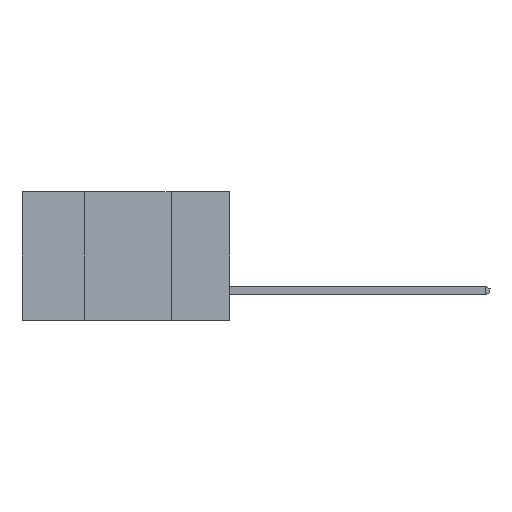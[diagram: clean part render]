
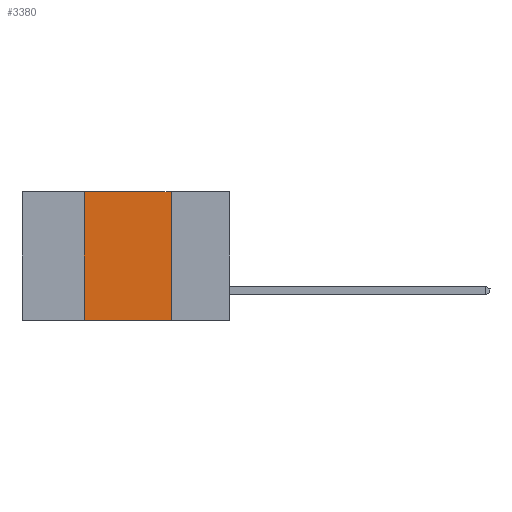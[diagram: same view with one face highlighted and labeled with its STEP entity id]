
A CAD part, left-side view. The second image highlights one B-rep face of the part: STEP entity #3380.
In plain terms, the highlighted planar face has unit normal (-1, 0, 0).
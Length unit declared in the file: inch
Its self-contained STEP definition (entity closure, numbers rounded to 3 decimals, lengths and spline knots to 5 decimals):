
#35 = CARTESIAN_POINT ( 'NONE',  ( 0., 0.42, -0.37 ) ) ;
#227 = ORIENTED_EDGE ( 'NONE', *, *, #5666, .F. ) ;
#707 = DIRECTION ( 'NONE',  ( 0., 0., -1. ) ) ;
#739 = AXIS2_PLACEMENT_3D ( 'NONE', #8256, #2847, #9026 ) ;
#811 = DIRECTION ( 'NONE',  ( 0., -1., 0. ) ) ;
#896 = CARTESIAN_POINT ( 'NONE',  ( 0., 0.17, -0.37 ) ) ;
#1425 = LINE ( 'NONE', #6782, #7478 ) ;
#2050 = ORIENTED_EDGE ( 'NONE', *, *, #7168, .F. ) ;
#2222 = EDGE_CURVE ( 'NONE', #7654, #8650, #4443, .T. ) ;
#2847 = DIRECTION ( 'NONE',  ( 1., 0., 0. ) ) ;
#3380 = ADVANCED_FACE ( 'NONE', ( #6602 ), #8207, .F. ) ;
#4443 = LINE ( 'NONE', #9164, #8667 ) ;
#4471 = DIRECTION ( 'NONE',  ( 0., 0., 1. ) ) ;
#5181 = EDGE_CURVE ( 'NONE', #6304, #8650, #1425, .T. ) ;
#5288 = CARTESIAN_POINT ( 'NONE',  ( 0., 0.42, -0.37 ) ) ;
#5294 = EDGE_LOOP ( 'NONE', ( #7462, #2050, #227, #6619 ) ) ;
#5495 = CARTESIAN_POINT ( 'NONE',  ( 0., 0.42, 0. ) ) ;
#5666 = EDGE_CURVE ( 'NONE', #7654, #7125, #8377, .T. ) ;
#6185 = CARTESIAN_POINT ( 'NONE',  ( 0., 0.6, 0. ) ) ;
#6304 = VERTEX_POINT ( 'NONE', #9864 ) ;
#6564 = VECTOR ( 'NONE', #9270, 39.37008 ) ;
#6602 = FACE_OUTER_BOUND ( 'NONE', #5294, .T. ) ;
#6619 = ORIENTED_EDGE ( 'NONE', *, *, #2222, .T. ) ;
#6782 = CARTESIAN_POINT ( 'NONE',  ( 0., 0.17, -0.37 ) ) ;
#7125 = VERTEX_POINT ( 'NONE', #5495 ) ;
#7168 = EDGE_CURVE ( 'NONE', #7125, #6304, #8457, .T. ) ;
#7462 = ORIENTED_EDGE ( 'NONE', *, *, #5181, .F. ) ;
#7478 = VECTOR ( 'NONE', #707, 39.37008 ) ;
#7634 = VECTOR ( 'NONE', #4471, 39.37008 ) ;
#7654 = VERTEX_POINT ( 'NONE', #5288 ) ;
#8207 = PLANE ( 'NONE',  #739 ) ;
#8256 = CARTESIAN_POINT ( 'NONE',  ( 0., 0.6, 0. ) ) ;
#8377 = LINE ( 'NONE', #35, #7634 ) ;
#8457 = LINE ( 'NONE', #6185, #6564 ) ;
#8650 = VERTEX_POINT ( 'NONE', #896 ) ;
#8667 = VECTOR ( 'NONE', #811, 39.37008 ) ;
#9026 = DIRECTION ( 'NONE',  ( 0., 0., -1. ) ) ;
#9164 = CARTESIAN_POINT ( 'NONE',  ( 0., 0.6, -0.37 ) ) ;
#9270 = DIRECTION ( 'NONE',  ( 0., -1., 0. ) ) ;
#9864 = CARTESIAN_POINT ( 'NONE',  ( 0., 0.17, 0. ) ) ;
